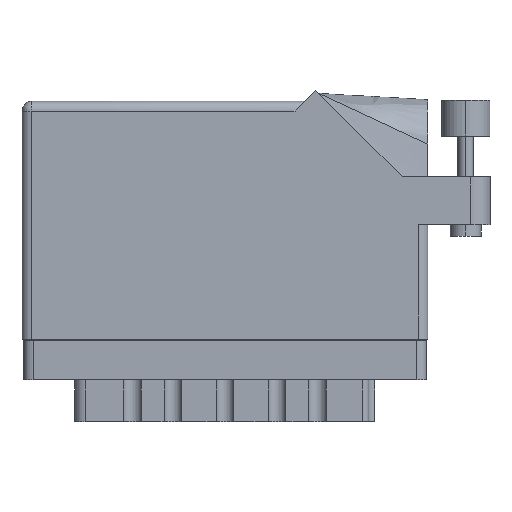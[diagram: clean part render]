
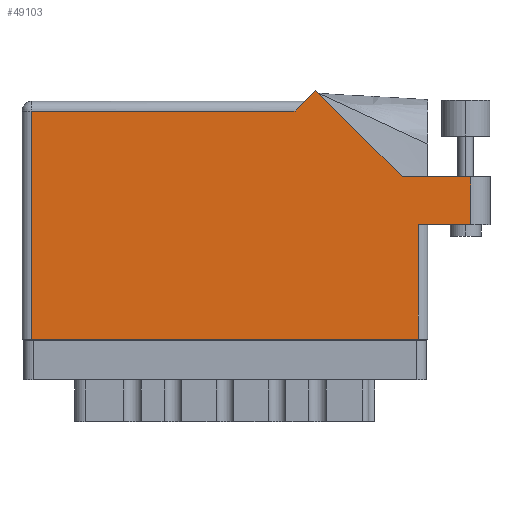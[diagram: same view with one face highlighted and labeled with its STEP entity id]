
A CAD part, front view. The second image highlights one B-rep face of the part: STEP entity #49103.
In plain terms, the highlighted face is planar.
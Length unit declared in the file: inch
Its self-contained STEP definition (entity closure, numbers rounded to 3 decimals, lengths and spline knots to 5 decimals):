
#1493 = ORIENTED_EDGE ( 'NONE', *, *, #12440, .T. ) ;
#3712 = VECTOR ( 'NONE', #12268, 39.37008 ) ;
#6762 = CARTESIAN_POINT ( 'NONE',  ( 1.819, 1.53, 0. ) ) ;
#7205 = CARTESIAN_POINT ( 'NONE',  ( 2.887, 1.044, 0. ) ) ;
#7406 = VERTEX_POINT ( 'NONE', #32626 ) ;
#7814 = DIRECTION ( 'NONE',  ( -0.707, -0.707, 0. ) ) ;
#8119 = DIRECTION ( 'NONE',  ( 0., 1., 0. ) ) ;
#8186 = EDGE_CURVE ( 'NONE', #13073, #7406, #44980, .T. ) ;
#8208 = DIRECTION ( 'NONE',  ( 0., 0., -1. ) ) ;
#9665 = VECTOR ( 'NONE', #16707, 39.37008 ) ;
#9972 = DIRECTION ( 'NONE',  ( 1., 0., 0. ) ) ;
#11385 = CARTESIAN_POINT ( 'NONE',  ( 0., 0., 0. ) ) ;
#11623 = CARTESIAN_POINT ( 'NONE',  ( 2.44642, 1.044, 0. ) ) ;
#11930 = VERTEX_POINT ( 'NONE', #40596 ) ;
#12268 = DIRECTION ( 'NONE',  ( -0.707, 0.707, 0. ) ) ;
#12440 = EDGE_CURVE ( 'NONE', #16851, #41912, #32004, .T. ) ;
#12663 = ORIENTED_EDGE ( 'NONE', *, *, #8186, .T. ) ;
#13073 = VERTEX_POINT ( 'NONE', #34526 ) ;
#13497 = CARTESIAN_POINT ( 'NONE',  ( 2.612, 0.737, 0. ) ) ;
#13607 = VECTOR ( 'NONE', #9972, 39.37008 ) ;
#14048 = VECTOR ( 'NONE', #7814, 39.37008 ) ;
#16707 = DIRECTION ( 'NONE',  ( 0., -1., 0. ) ) ;
#16851 = VERTEX_POINT ( 'NONE', #21290 ) ;
#17146 = CARTESIAN_POINT ( 'NONE',  ( 2.55, 0.737, 0. ) ) ;
#17770 = EDGE_CURVE ( 'NONE', #25050, #39110, #40960, .T. ) ;
#18436 = LINE ( 'NONE', #41662, #9665 ) ;
#19019 = CARTESIAN_POINT ( 'NONE',  ( 2.887, 1.044, 0. ) ) ;
#20184 = CARTESIAN_POINT ( 'NONE',  ( 2.55, 0., 0. ) ) ;
#20561 = VERTEX_POINT ( 'NONE', #17146 ) ;
#21290 = CARTESIAN_POINT ( 'NONE',  ( 0.062, 0., 0. ) ) ;
#21608 = VECTOR ( 'NONE', #31731, 39.37008 ) ;
#21882 = VECTOR ( 'NONE', #48985, 39.37008 ) ;
#22042 = ORIENTED_EDGE ( 'NONE', *, *, #36404, .T. ) ;
#23463 = EDGE_LOOP ( 'NONE', ( #41186, #50539, #45464, #34395, #12663, #53558, #39983, #1493, #22042 ) ) ;
#23654 = VECTOR ( 'NONE', #48855, 39.37008 ) ;
#24079 = EDGE_CURVE ( 'NONE', #39110, #13073, #33426, .T. ) ;
#24527 = AXIS2_PLACEMENT_3D ( 'NONE', #45369, #8208, #24725 ) ;
#24725 = DIRECTION ( 'NONE',  ( -1., 0., 0. ) ) ;
#24793 = CARTESIAN_POINT ( 'NONE',  ( 0., 1.468, 0. ) ) ;
#25050 = VERTEX_POINT ( 'NONE', #7205 ) ;
#27346 = CARTESIAN_POINT ( 'NONE',  ( 0.062, 1.468, 0. ) ) ;
#27429 = LINE ( 'NONE', #19019, #51577 ) ;
#28283 = VERTEX_POINT ( 'NONE', #27346 ) ;
#28796 = FACE_OUTER_BOUND ( 'NONE', #23463, .T. ) ;
#28983 = CARTESIAN_POINT ( 'NONE',  ( 2.55, 0.737, 0. ) ) ;
#31731 = DIRECTION ( 'NONE',  ( 1., 0., 0. ) ) ;
#32004 = LINE ( 'NONE', #11385, #21608 ) ;
#32626 = CARTESIAN_POINT ( 'NONE',  ( 1.757, 1.468, 0. ) ) ;
#32793 = VECTOR ( 'NONE', #8119, 39.37008 ) ;
#33090 = EDGE_CURVE ( 'NONE', #11930, #25050, #27429, .T. ) ;
#33426 = LINE ( 'NONE', #49438, #3712 ) ;
#34395 = ORIENTED_EDGE ( 'NONE', *, *, #24079, .T. ) ;
#34526 = CARTESIAN_POINT ( 'NONE',  ( 1.88971, 1.60071, 0. ) ) ;
#34655 = LINE ( 'NONE', #13497, #13607 ) ;
#35257 = EDGE_CURVE ( 'NONE', #20561, #11930, #34655, .T. ) ;
#35314 = DIRECTION ( 'NONE',  ( 0., 1., 0. ) ) ;
#36404 = EDGE_CURVE ( 'NONE', #41912, #20561, #45552, .T. ) ;
#39110 = VERTEX_POINT ( 'NONE', #11623 ) ;
#39983 = ORIENTED_EDGE ( 'NONE', *, *, #47495, .T. ) ;
#40596 = CARTESIAN_POINT ( 'NONE',  ( 2.887, 0.737, 0. ) ) ;
#40960 = LINE ( 'NONE', #52671, #23654 ) ;
#41186 = ORIENTED_EDGE ( 'NONE', *, *, #35257, .T. ) ;
#41662 = CARTESIAN_POINT ( 'NONE',  ( 0.062, 0., 0. ) ) ;
#41912 = VERTEX_POINT ( 'NONE', #20184 ) ;
#44980 = LINE ( 'NONE', #6762, #14048 ) ;
#45165 = LINE ( 'NONE', #24793, #21882 ) ;
#45369 = CARTESIAN_POINT ( 'NONE',  ( 0., 1.53, 0. ) ) ;
#45464 = ORIENTED_EDGE ( 'NONE', *, *, #17770, .T. ) ;
#45552 = LINE ( 'NONE', #28983, #32793 ) ;
#47495 = EDGE_CURVE ( 'NONE', #28283, #16851, #18436, .T. ) ;
#48615 = EDGE_CURVE ( 'NONE', #7406, #28283, #45165, .T. ) ;
#48855 = DIRECTION ( 'NONE',  ( -1., 0., 0. ) ) ;
#48985 = DIRECTION ( 'NONE',  ( -1., 0., 0. ) ) ;
#49103 = ADVANCED_FACE ( 'NONE', ( #28796 ), #52985, .F. ) ;
#49438 = CARTESIAN_POINT ( 'NONE',  ( 2.44642, 1.044, 0. ) ) ;
#50539 = ORIENTED_EDGE ( 'NONE', *, *, #33090, .T. ) ;
#51577 = VECTOR ( 'NONE', #35314, 39.37008 ) ;
#52671 = CARTESIAN_POINT ( 'NONE',  ( 3.012, 1.044, 0. ) ) ;
#52985 = PLANE ( 'NONE',  #24527 ) ;
#53558 = ORIENTED_EDGE ( 'NONE', *, *, #48615, .T. ) ;
